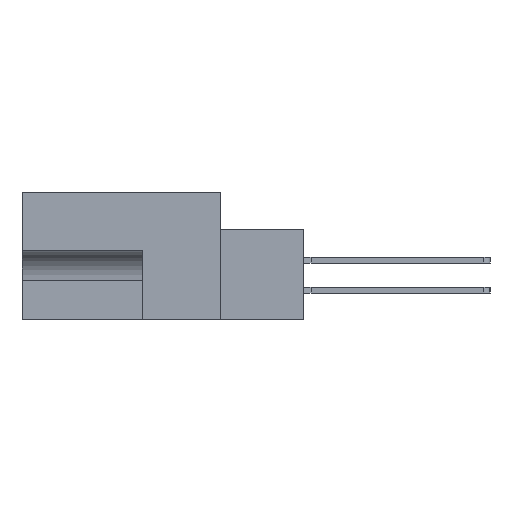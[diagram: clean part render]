
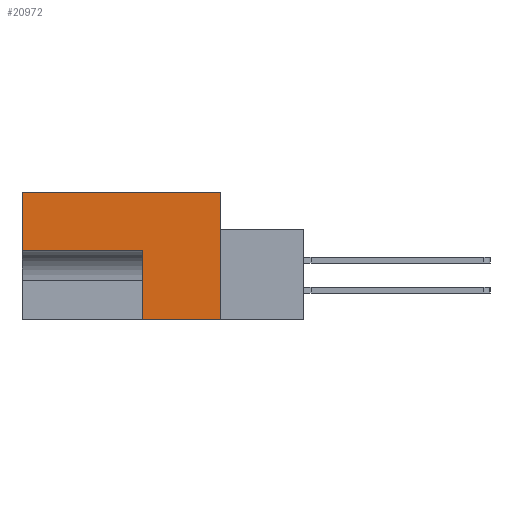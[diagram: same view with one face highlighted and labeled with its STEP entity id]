
A CAD part, left-side view. The second image highlights one B-rep face of the part: STEP entity #20972.
In plain terms, the highlighted planar face has unit normal (-1, 0, 0).
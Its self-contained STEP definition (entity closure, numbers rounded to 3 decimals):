
#1 = VECTOR ( 'NONE', #31035, 1000. ) ;
#207 = CARTESIAN_POINT ( 'NONE',  ( 0., 0., 0. ) ) ;
#2215 = ORIENTED_EDGE ( 'NONE', *, *, #32934, .F. ) ;
#2397 = ORIENTED_EDGE ( 'NONE', *, *, #46042, .F. ) ;
#2647 = DIRECTION ( 'NONE',  ( 0., 1., 0. ) ) ;
#3139 = ORIENTED_EDGE ( 'NONE', *, *, #35172, .F. ) ;
#5109 = LINE ( 'NONE', #41172, #29126 ) ;
#5379 = VERTEX_POINT ( 'NONE', #32230 ) ;
#7373 = CARTESIAN_POINT ( 'NONE',  ( 0., 20.955, -6.172 ) ) ;
#7860 = CARTESIAN_POINT ( 'NONE',  ( 0., 20.955, 0. ) ) ;
#8233 = EDGE_CURVE ( 'NONE', #27846, #33715, #5109, .T. ) ;
#8345 = DIRECTION ( 'NONE',  ( 0., 1., 0. ) ) ;
#8905 = CARTESIAN_POINT ( 'NONE',  ( 0., 0., -13.487 ) ) ;
#9541 = VERTEX_POINT ( 'NONE', #7373 ) ;
#10720 = CARTESIAN_POINT ( 'NONE',  ( 0., 20.955, -13.487 ) ) ;
#10855 = CARTESIAN_POINT ( 'NONE',  ( 0., -8.814, -13.487 ) ) ;
#12374 = CARTESIAN_POINT ( 'NONE',  ( 0., 0., 0. ) ) ;
#18840 = LINE ( 'NONE', #37149, #41169 ) ;
#19329 = DIRECTION ( 'NONE',  ( 0., 0., 1. ) ) ;
#19840 = VERTEX_POINT ( 'NONE', #8905 ) ;
#20470 = CARTESIAN_POINT ( 'NONE',  ( 0., 8.255, -6.172 ) ) ;
#20972 = ADVANCED_FACE ( 'NONE', ( #39931 ), #22990, .F. ) ;
#21752 = LINE ( 'NONE', #35124, #1 ) ;
#22987 = ORIENTED_EDGE ( 'NONE', *, *, #42568, .F. ) ;
#22990 = PLANE ( 'NONE',  #24053 ) ;
#24053 = AXIS2_PLACEMENT_3D ( 'NONE', #12374, #37549, #37394 ) ;
#24335 = EDGE_CURVE ( 'NONE', #5379, #9541, #43755, .T. ) ;
#25272 = EDGE_LOOP ( 'NONE', ( #22987, #3139, #42633, #2215, #27513, #2397 ) ) ;
#27513 = ORIENTED_EDGE ( 'NONE', *, *, #24335, .F. ) ;
#27846 = VERTEX_POINT ( 'NONE', #7860 ) ;
#28998 = DIRECTION ( 'NONE',  ( 0., 0., 1. ) ) ;
#29126 = VECTOR ( 'NONE', #30706, 1000. ) ;
#29225 = VECTOR ( 'NONE', #2647, 1000. ) ;
#30706 = DIRECTION ( 'NONE',  ( 0., -1., 0. ) ) ;
#31035 = DIRECTION ( 'NONE',  ( 0., 0., -1. ) ) ;
#31148 = VECTOR ( 'NONE', #28998, 1000. ) ;
#32199 = CARTESIAN_POINT ( 'NONE',  ( 0., 8.255, -13.487 ) ) ;
#32230 = CARTESIAN_POINT ( 'NONE',  ( 0., 8.255, -6.172 ) ) ;
#32833 = LINE ( 'NONE', #10855, #41209 ) ;
#32934 = EDGE_CURVE ( 'NONE', #9541, #27846, #40647, .T. ) ;
#33715 = VERTEX_POINT ( 'NONE', #207 ) ;
#35124 = CARTESIAN_POINT ( 'NONE',  ( 0., 0., 0. ) ) ;
#35172 = EDGE_CURVE ( 'NONE', #33715, #19840, #21752, .T. ) ;
#37149 = CARTESIAN_POINT ( 'NONE',  ( 0., 8.255, -13.487 ) ) ;
#37394 = DIRECTION ( 'NONE',  ( 0., 0., -1. ) ) ;
#37529 = VERTEX_POINT ( 'NONE', #32199 ) ;
#37549 = DIRECTION ( 'NONE',  ( 1., 0., 0. ) ) ;
#39931 = FACE_OUTER_BOUND ( 'NONE', #25272, .T. ) ;
#40647 = LINE ( 'NONE', #10720, #31148 ) ;
#41169 = VECTOR ( 'NONE', #19329, 1000. ) ;
#41172 = CARTESIAN_POINT ( 'NONE',  ( 0., 11.506, 0. ) ) ;
#41209 = VECTOR ( 'NONE', #8345, 1000. ) ;
#42568 = EDGE_CURVE ( 'NONE', #19840, #37529, #32833, .T. ) ;
#42633 = ORIENTED_EDGE ( 'NONE', *, *, #8233, .F. ) ;
#43755 = LINE ( 'NONE', #20470, #29225 ) ;
#46042 = EDGE_CURVE ( 'NONE', #37529, #5379, #18840, .T. ) ;
